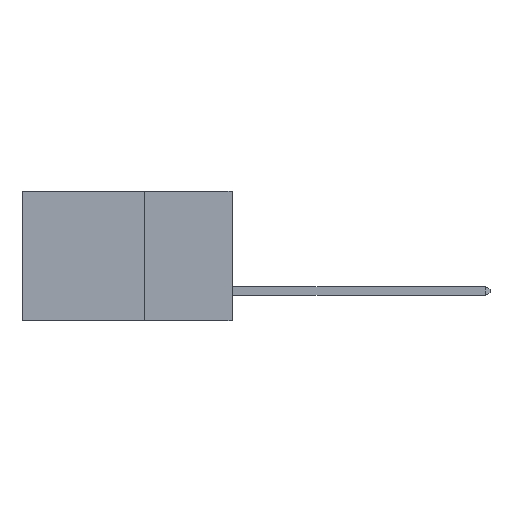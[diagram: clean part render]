
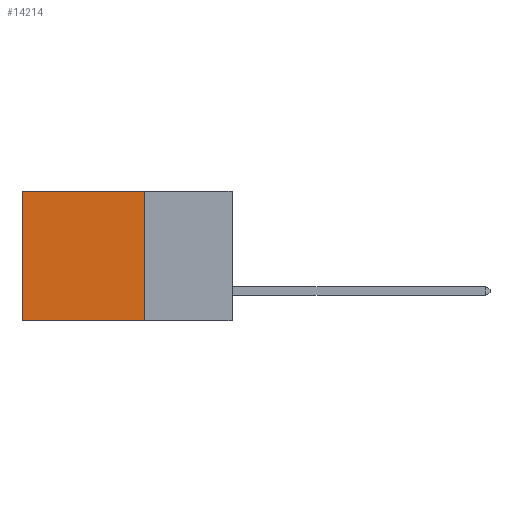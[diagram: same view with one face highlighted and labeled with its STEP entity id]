
A CAD part, left-side view. The second image highlights one B-rep face of the part: STEP entity #14214.
In plain terms, the highlighted planar face has unit normal (-1, 0, 0).
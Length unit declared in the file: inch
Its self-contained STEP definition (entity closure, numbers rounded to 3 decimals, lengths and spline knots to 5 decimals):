
#8 = CARTESIAN_POINT ( 'NONE',  ( 0.2875, 0.25, 0. ) ) ;
#1419 = VECTOR ( 'NONE', #1466, 39.37008 ) ;
#1466 = DIRECTION ( 'NONE',  ( 0., 0., -1. ) ) ;
#2091 = VERTEX_POINT ( 'NONE', #18373 ) ;
#2206 = DIRECTION ( 'NONE',  ( 1., 0., 0. ) ) ;
#2898 = AXIS2_PLACEMENT_3D ( 'NONE', #8, #2206, #16912 ) ;
#3402 = EDGE_CURVE ( 'NONE', #19621, #14414, #9248, .T. ) ;
#3625 = VERTEX_POINT ( 'NONE', #16960 ) ;
#3883 = VECTOR ( 'NONE', #14989, 39.37008 ) ;
#4430 = ORIENTED_EDGE ( 'NONE', *, *, #26047, .T. ) ;
#6958 = VECTOR ( 'NONE', #8484, 39.37008 ) ;
#7279 = EDGE_CURVE ( 'NONE', #3625, #14414, #18198, .T. ) ;
#8484 = DIRECTION ( 'NONE',  ( 0., 0., -1. ) ) ;
#9248 = LINE ( 'NONE', #14216, #15462 ) ;
#12698 = PLANE ( 'NONE',  #2898 ) ;
#14214 = ADVANCED_FACE ( 'NONE', ( #17184 ), #12698, .F. ) ;
#14216 = CARTESIAN_POINT ( 'NONE',  ( 0.2875, 0.25, -0.37 ) ) ;
#14414 = VERTEX_POINT ( 'NONE', #17543 ) ;
#14988 = LINE ( 'NONE', #25435, #3883 ) ;
#14989 = DIRECTION ( 'NONE',  ( 0., 1., 0. ) ) ;
#15112 = ORIENTED_EDGE ( 'NONE', *, *, #7279, .T. ) ;
#15462 = VECTOR ( 'NONE', #22539, 39.37008 ) ;
#16489 = CARTESIAN_POINT ( 'NONE',  ( 0.2875, 0.25, -0.37 ) ) ;
#16912 = DIRECTION ( 'NONE',  ( 0., 0., -1. ) ) ;
#16960 = CARTESIAN_POINT ( 'NONE',  ( 0.2875, 0.6, 0. ) ) ;
#17184 = FACE_OUTER_BOUND ( 'NONE', #18064, .T. ) ;
#17543 = CARTESIAN_POINT ( 'NONE',  ( 0.2875, 0.6, -0.37 ) ) ;
#17564 = ORIENTED_EDGE ( 'NONE', *, *, #3402, .F. ) ;
#18064 = EDGE_LOOP ( 'NONE', ( #15112, #17564, #22742, #4430 ) ) ;
#18198 = LINE ( 'NONE', #22389, #1419 ) ;
#18373 = CARTESIAN_POINT ( 'NONE',  ( 0.2875, 0.25, 0. ) ) ;
#18461 = EDGE_CURVE ( 'NONE', #2091, #19621, #23666, .T. ) ;
#19621 = VERTEX_POINT ( 'NONE', #16489 ) ;
#22389 = CARTESIAN_POINT ( 'NONE',  ( 0.2875, 0.6, 0. ) ) ;
#22539 = DIRECTION ( 'NONE',  ( 0., 1., 0. ) ) ;
#22742 = ORIENTED_EDGE ( 'NONE', *, *, #18461, .F. ) ;
#23666 = LINE ( 'NONE', #25230, #6958 ) ;
#25230 = CARTESIAN_POINT ( 'NONE',  ( 0.2875, 0.25, 0. ) ) ;
#25435 = CARTESIAN_POINT ( 'NONE',  ( 0.2875, 0.25, 0. ) ) ;
#26047 = EDGE_CURVE ( 'NONE', #2091, #3625, #14988, .T. ) ;
